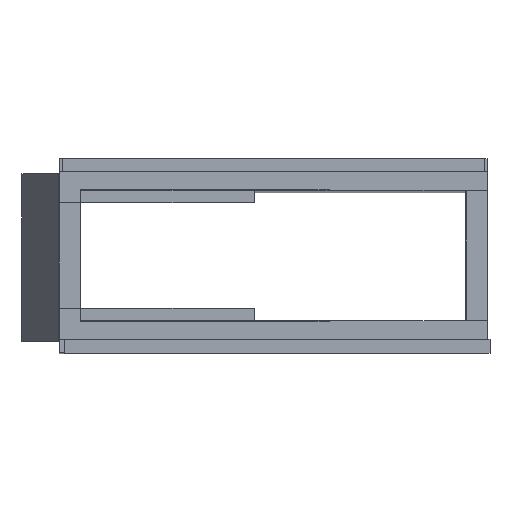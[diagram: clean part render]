
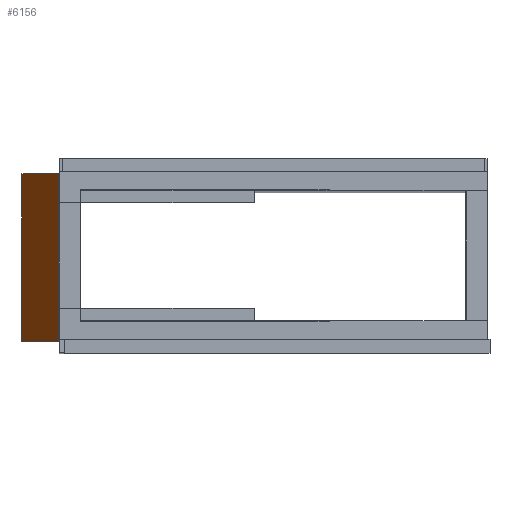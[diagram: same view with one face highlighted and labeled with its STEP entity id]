
A CAD part, top view. The second image highlights one B-rep face of the part: STEP entity #6156.
In plain terms, the highlighted planar face has unit normal (-0.955, 0, 0.297).
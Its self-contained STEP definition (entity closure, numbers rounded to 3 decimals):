
#1116 = PLANE('',#1117);
#1117 = AXIS2_PLACEMENT_3D('',#1118,#1119,#1120);
#1118 = CARTESIAN_POINT('',(-34.45,13.5,25.));
#1119 = DIRECTION('',(0.,1.,0.));
#1120 = DIRECTION('',(0.,0.,1.));
#2640 = PLANE('',#2641);
#2641 = AXIS2_PLACEMENT_3D('',#2642,#2643,#2644);
#2642 = CARTESIAN_POINT('',(-34.45,0.,25.));
#2643 = DIRECTION('',(0.,0.,-1.));
#2644 = DIRECTION('',(0.,1.,0.));
#2936 = VERTEX_POINT('',#2937);
#2937 = CARTESIAN_POINT('',(-37.431,13.5,25.));
#2958 = EDGE_CURVE('',#2959,#2936,#2961,.T.);
#2959 = VERTEX_POINT('',#2960);
#2960 = CARTESIAN_POINT('',(-34.495,13.5,34.445));
#2961 = SURFACE_CURVE('',#2962,(#2966,#2973),.PCURVE_S1.);
#2962 = LINE('',#2963,#2964);
#2963 = CARTESIAN_POINT('',(-34.474,13.5,34.512));
#2964 = VECTOR('',#2965,1.);
#2965 = DIRECTION('',(-0.297,0.,
    -0.955));
#2966 = PCURVE('',#1116,#2967);
#2967 = DEFINITIONAL_REPRESENTATION('',(#2968),#2972);
#2968 = LINE('',#2969,#2970);
#2969 = CARTESIAN_POINT('',(9.512,-0.024));
#2970 = VECTOR('',#2971,1.);
#2971 = DIRECTION('',(-0.955,-0.297));
#2972 = ( GEOMETRIC_REPRESENTATION_CONTEXT(2) 
PARAMETRIC_REPRESENTATION_CONTEXT() REPRESENTATION_CONTEXT('2D SPACE',''
  ) );
#2973 = PCURVE('',#2974,#2979);
#2974 = PLANE('',#2975);
#2975 = AXIS2_PLACEMENT_3D('',#2976,#2977,#2978);
#2976 = CARTESIAN_POINT('',(-34.474,13.5,34.512));
#2977 = DIRECTION('',(0.955,0.,
    -0.297));
#2978 = DIRECTION('',(-0.297,0.,
    -0.955));
#2979 = DEFINITIONAL_REPRESENTATION('',(#2980),#2984);
#2980 = LINE('',#2981,#2982);
#2981 = CARTESIAN_POINT('',(0.,0.));
#2982 = VECTOR('',#2983,1.);
#2983 = DIRECTION('',(1.,0.));
#2984 = ( GEOMETRIC_REPRESENTATION_CONTEXT(2) 
PARAMETRIC_REPRESENTATION_CONTEXT() REPRESENTATION_CONTEXT('2D SPACE',''
  ) );
#3000 = PLANE('',#3001);
#3001 = AXIS2_PLACEMENT_3D('',#3002,#3003,#3004);
#3002 = CARTESIAN_POINT('',(-34.45,13.5,34.445));
#3003 = DIRECTION('',(0.,0.,1.));
#3004 = DIRECTION('',(0.,-1.,0.));
#3684 = PLANE('',#3685);
#3685 = AXIS2_PLACEMENT_3D('',#3686,#3687,#3688);
#3686 = CARTESIAN_POINT('',(-34.45,0.,34.445));
#3687 = DIRECTION('',(0.,-1.,0.));
#3688 = DIRECTION('',(0.,0.,-1.));
#5792 = EDGE_CURVE('',#2936,#5793,#5795,.T.);
#5793 = VERTEX_POINT('',#5794);
#5794 = CARTESIAN_POINT('',(-37.431,0.,25.));
#5795 = SURFACE_CURVE('',#5796,(#5800,#5806),.PCURVE_S1.);
#5796 = LINE('',#5797,#5798);
#5797 = CARTESIAN_POINT('',(-37.431,6.75,25.));
#5798 = VECTOR('',#5799,1.);
#5799 = DIRECTION('',(0.,-1.,0.));
#5800 = PCURVE('',#2640,#5801);
#5801 = DEFINITIONAL_REPRESENTATION('',(#5802),#5805);
#5802 = B_SPLINE_CURVE_WITH_KNOTS('',1,(#5803,#5804),.UNSPECIFIED.,.F.,
  .F.,(2,2),(-6.75,6.75),.PIECEWISE_BEZIER_KNOTS.);
#5803 = CARTESIAN_POINT('',(13.5,-2.981));
#5804 = CARTESIAN_POINT('',(0.,-2.981));
#5805 = ( GEOMETRIC_REPRESENTATION_CONTEXT(2) 
PARAMETRIC_REPRESENTATION_CONTEXT() REPRESENTATION_CONTEXT('2D SPACE',''
  ) );
#5806 = PCURVE('',#2974,#5807);
#5807 = DEFINITIONAL_REPRESENTATION('',(#5808),#5811);
#5808 = B_SPLINE_CURVE_WITH_KNOTS('',1,(#5809,#5810),.UNSPECIFIED.,.F.,
  .F.,(2,2),(-6.75,6.75),.PIECEWISE_BEZIER_KNOTS.);
#5809 = CARTESIAN_POINT('',(9.962,0.));
#5810 = CARTESIAN_POINT('',(9.962,-13.5));
#5811 = ( GEOMETRIC_REPRESENTATION_CONTEXT(2) 
PARAMETRIC_REPRESENTATION_CONTEXT() REPRESENTATION_CONTEXT('2D SPACE',''
  ) );
#6113 = EDGE_CURVE('',#6114,#2959,#6116,.T.);
#6114 = VERTEX_POINT('',#6115);
#6115 = CARTESIAN_POINT('',(-34.495,0.,34.445));
#6116 = SURFACE_CURVE('',#6117,(#6121,#6127),.PCURVE_S1.);
#6117 = LINE('',#6118,#6119);
#6118 = CARTESIAN_POINT('',(-34.495,13.5,34.445));
#6119 = VECTOR('',#6120,1.);
#6120 = DIRECTION('',(0.,1.,0.));
#6121 = PCURVE('',#3000,#6122);
#6122 = DEFINITIONAL_REPRESENTATION('',(#6123),#6126);
#6123 = B_SPLINE_CURVE_WITH_KNOTS('',1,(#6124,#6125),.UNSPECIFIED.,.F.,
  .F.,(2,2),(-13.5,0.),.PIECEWISE_BEZIER_KNOTS.);
#6124 = CARTESIAN_POINT('',(13.5,-0.045));
#6125 = CARTESIAN_POINT('',(0.,-0.045));
#6126 = ( GEOMETRIC_REPRESENTATION_CONTEXT(2) 
PARAMETRIC_REPRESENTATION_CONTEXT() REPRESENTATION_CONTEXT('2D SPACE',''
  ) );
#6127 = PCURVE('',#2974,#6128);
#6128 = DEFINITIONAL_REPRESENTATION('',(#6129),#6132);
#6129 = B_SPLINE_CURVE_WITH_KNOTS('',1,(#6130,#6131),.UNSPECIFIED.,.F.,
  .F.,(2,2),(-13.5,0.),.PIECEWISE_BEZIER_KNOTS.);
#6130 = CARTESIAN_POINT('',(0.071,-13.5));
#6131 = CARTESIAN_POINT('',(0.071,0.));
#6132 = ( GEOMETRIC_REPRESENTATION_CONTEXT(2) 
PARAMETRIC_REPRESENTATION_CONTEXT() REPRESENTATION_CONTEXT('2D SPACE',''
  ) );
#6156 = ADVANCED_FACE('',(#6157),#2974,.F.);
#6157 = FACE_BOUND('',#6158,.F.);
#6158 = EDGE_LOOP('',(#6159,#6160,#6161,#6162));
#6159 = ORIENTED_EDGE('',*,*,#5792,.F.);
#6160 = ORIENTED_EDGE('',*,*,#2958,.F.);
#6161 = ORIENTED_EDGE('',*,*,#6113,.F.);
#6162 = ORIENTED_EDGE('',*,*,#6163,.F.);
#6163 = EDGE_CURVE('',#5793,#6114,#6164,.T.);
#6164 = SURFACE_CURVE('',#6165,(#6169,#6175),.PCURVE_S1.);
#6165 = LINE('',#6166,#6167);
#6166 = CARTESIAN_POINT('',(-34.482,0.,34.485));
#6167 = VECTOR('',#6168,1.);
#6168 = DIRECTION('',(0.297,0.,0.955));
#6169 = PCURVE('',#2974,#6170);
#6170 = DEFINITIONAL_REPRESENTATION('',(#6171),#6174);
#6171 = B_SPLINE_CURVE_WITH_KNOTS('',1,(#6172,#6173),.UNSPECIFIED.,.F.,
  .F.,(2,2),(-9.933,-0.042),
  .PIECEWISE_BEZIER_KNOTS.);
#6172 = CARTESIAN_POINT('',(9.962,-13.5));
#6173 = CARTESIAN_POINT('',(0.071,-13.5));
#6174 = ( GEOMETRIC_REPRESENTATION_CONTEXT(2) 
PARAMETRIC_REPRESENTATION_CONTEXT() REPRESENTATION_CONTEXT('2D SPACE',''
  ) );
#6175 = PCURVE('',#3684,#6176);
#6176 = DEFINITIONAL_REPRESENTATION('',(#6177),#6180);
#6177 = B_SPLINE_CURVE_WITH_KNOTS('',1,(#6178,#6179),.UNSPECIFIED.,.F.,
  .F.,(2,2),(-9.933,-0.042),
  .PIECEWISE_BEZIER_KNOTS.);
#6178 = CARTESIAN_POINT('',(9.445,-2.981));
#6179 = CARTESIAN_POINT('',(0.,-0.045));
#6180 = ( GEOMETRIC_REPRESENTATION_CONTEXT(2) 
PARAMETRIC_REPRESENTATION_CONTEXT() REPRESENTATION_CONTEXT('2D SPACE',''
  ) );
